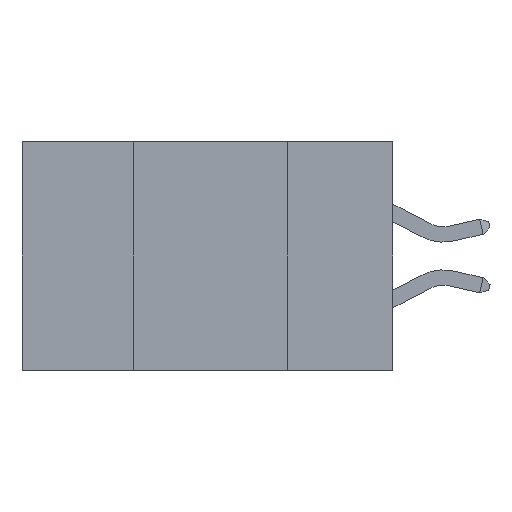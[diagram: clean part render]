
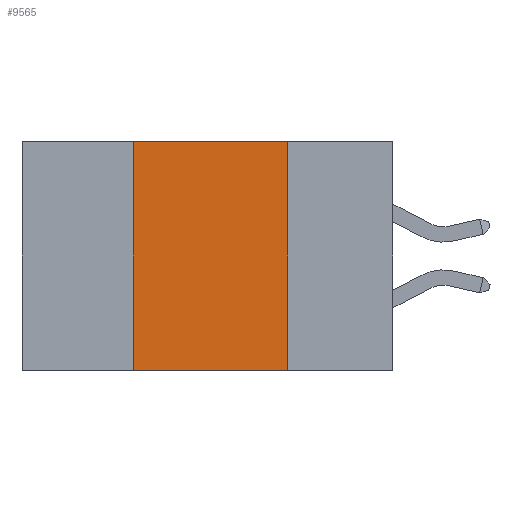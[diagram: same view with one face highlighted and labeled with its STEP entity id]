
A CAD part, left-side view. The second image highlights one B-rep face of the part: STEP entity #9565.
In plain terms, the highlighted planar face has unit normal (-1, 0, 0).
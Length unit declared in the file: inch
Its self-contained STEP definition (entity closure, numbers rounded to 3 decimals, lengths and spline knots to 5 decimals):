
#297 = DIRECTION ( 'NONE',  ( 1., 0., 0. ) ) ;
#428 = CARTESIAN_POINT ( 'NONE',  ( 0., 0.42, 0. ) ) ;
#475 = DIRECTION ( 'NONE',  ( 0., 0., -1. ) ) ;
#702 = EDGE_CURVE ( 'NONE', #13286, #3297, #6888, .T. ) ;
#1348 = EDGE_LOOP ( 'NONE', ( #3341, #12117, #4037, #10060 ) ) ;
#1647 = CARTESIAN_POINT ( 'NONE',  ( 0., 0.6, -0.37 ) ) ;
#1692 = LINE ( 'NONE', #1647, #7115 ) ;
#1851 = CARTESIAN_POINT ( 'NONE',  ( 0., 0.42, 0. ) ) ;
#3297 = VERTEX_POINT ( 'NONE', #428 ) ;
#3341 = ORIENTED_EDGE ( 'NONE', *, *, #13035, .F. ) ;
#4037 = ORIENTED_EDGE ( 'NONE', *, *, #702, .F. ) ;
#4326 = FACE_OUTER_BOUND ( 'NONE', #1348, .T. ) ;
#4426 = CARTESIAN_POINT ( 'NONE',  ( 0., 0.6, 0. ) ) ;
#4579 = VECTOR ( 'NONE', #12834, 39.37008 ) ;
#4791 = DIRECTION ( 'NONE',  ( 0., 0., 1. ) ) ;
#4890 = LINE ( 'NONE', #8024, #13576 ) ;
#5604 = EDGE_CURVE ( 'NONE', #3297, #8653, #7460, .T. ) ;
#5693 = PLANE ( 'NONE',  #11180 ) ;
#6888 = LINE ( 'NONE', #1851, #12063 ) ;
#7115 = VECTOR ( 'NONE', #8092, 39.37008 ) ;
#7460 = LINE ( 'NONE', #4426, #4579 ) ;
#7840 = DIRECTION ( 'NONE',  ( 0., 0., -1. ) ) ;
#7947 = CARTESIAN_POINT ( 'NONE',  ( 0., 0.17, -0.37 ) ) ;
#8024 = CARTESIAN_POINT ( 'NONE',  ( 0., 0.17, 0. ) ) ;
#8092 = DIRECTION ( 'NONE',  ( 0., -1., 0. ) ) ;
#8653 = VERTEX_POINT ( 'NONE', #10606 ) ;
#9565 = ADVANCED_FACE ( 'NONE', ( #4326 ), #5693, .F. ) ;
#10060 = ORIENTED_EDGE ( 'NONE', *, *, #13284, .T. ) ;
#10606 = CARTESIAN_POINT ( 'NONE',  ( 0., 0.17, 0. ) ) ;
#11180 = AXIS2_PLACEMENT_3D ( 'NONE', #12990, #297, #7840 ) ;
#12063 = VECTOR ( 'NONE', #4791, 39.37008 ) ;
#12117 = ORIENTED_EDGE ( 'NONE', *, *, #5604, .F. ) ;
#12368 = VERTEX_POINT ( 'NONE', #7947 ) ;
#12834 = DIRECTION ( 'NONE',  ( 0., -1., 0. ) ) ;
#12990 = CARTESIAN_POINT ( 'NONE',  ( 0., 0.6, 0. ) ) ;
#13035 = EDGE_CURVE ( 'NONE', #8653, #12368, #4890, .T. ) ;
#13284 = EDGE_CURVE ( 'NONE', #13286, #12368, #1692, .T. ) ;
#13286 = VERTEX_POINT ( 'NONE', #13607 ) ;
#13576 = VECTOR ( 'NONE', #475, 39.37008 ) ;
#13607 = CARTESIAN_POINT ( 'NONE',  ( 0., 0.42, -0.37 ) ) ;
